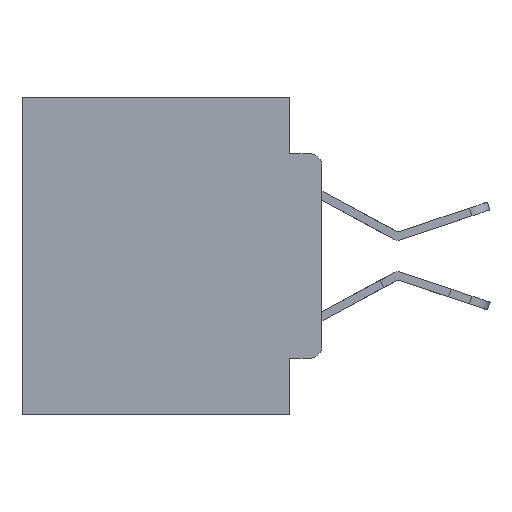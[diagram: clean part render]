
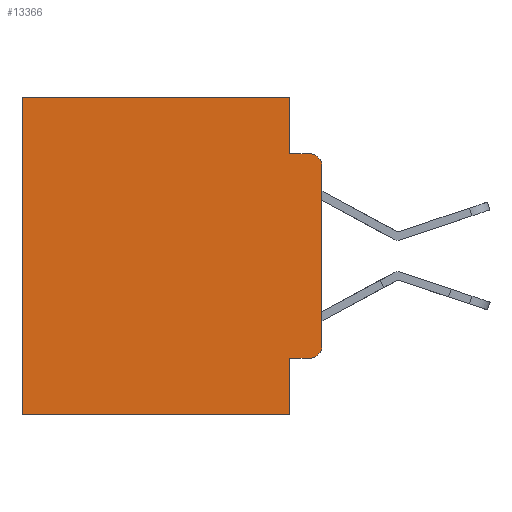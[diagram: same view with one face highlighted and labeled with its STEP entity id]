
A CAD part, left-side view. The second image highlights one B-rep face of the part: STEP entity #13366.
In plain terms, the highlighted planar face has unit normal (-1, 0, 0).
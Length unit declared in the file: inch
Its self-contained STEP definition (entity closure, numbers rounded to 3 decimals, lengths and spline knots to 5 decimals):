
#502 = LINE ( 'NONE', #6662, #24022 ) ;
#746 = VECTOR ( 'NONE', #17544, 39.37008 ) ;
#786 = CARTESIAN_POINT ( 'NONE',  ( 0.298, 0., -0.1085 ) ) ;
#980 = VERTEX_POINT ( 'NONE', #29795 ) ;
#1310 = EDGE_CURVE ( 'NONE', #6025, #29234, #16941, .T. ) ;
#1388 = DIRECTION ( 'NONE',  ( 0., 0., -1. ) ) ;
#1854 = LINE ( 'NONE', #29069, #21708 ) ;
#2882 = ORIENTED_EDGE ( 'NONE', *, *, #23041, .F. ) ;
#2899 = DIRECTION ( 'NONE',  ( 0., 0., -1. ) ) ;
#2971 = CARTESIAN_POINT ( 'NONE',  ( 0.298, 0.02, -0.1085 ) ) ;
#3745 = LINE ( 'NONE', #8295, #15320 ) ;
#3854 = PLANE ( 'NONE',  #16851 ) ;
#4271 = VERTEX_POINT ( 'NONE', #22467 ) ;
#4990 = DIRECTION ( 'NONE',  ( 0., -1., 0. ) ) ;
#5420 = VECTOR ( 'NONE', #11482, 39.37008 ) ;
#5625 = FACE_OUTER_BOUND ( 'NONE', #14080, .T. ) ;
#5909 = CARTESIAN_POINT ( 'NONE',  ( 0.298, 0., -0.5 ) ) ;
#6025 = VERTEX_POINT ( 'NONE', #17912 ) ;
#6082 = DIRECTION ( 'NONE',  ( -1., 0., 0. ) ) ;
#6245 = DIRECTION ( 'NONE',  ( 0., 0., -1. ) ) ;
#6429 = EDGE_CURVE ( 'NONE', #980, #21504, #19172, .T. ) ;
#6631 = EDGE_CURVE ( 'NONE', #27518, #980, #18816, .T. ) ;
#6662 = CARTESIAN_POINT ( 'NONE',  ( 0.298, 0., 0. ) ) ;
#7044 = EDGE_CURVE ( 'NONE', #4271, #11649, #13814, .T. ) ;
#7847 = ORIENTED_EDGE ( 'NONE', *, *, #16300, .F. ) ;
#8295 = CARTESIAN_POINT ( 'NONE',  ( 0.298, 0., 0. ) ) ;
#8607 = EDGE_CURVE ( 'NONE', #27518, #4271, #1854, .T. ) ;
#8631 = CARTESIAN_POINT ( 'NONE',  ( 0.298, 0.02, -0.3915 ) ) ;
#8725 = CARTESIAN_POINT ( 'NONE',  ( 0.298, 0., -0.3915 ) ) ;
#9327 = CARTESIAN_POINT ( 'NONE',  ( 0.298, 0.473, 0. ) ) ;
#10028 = ORIENTED_EDGE ( 'NONE', *, *, #6631, .F. ) ;
#10473 = VECTOR ( 'NONE', #4990, 39.37008 ) ;
#10656 = ORIENTED_EDGE ( 'NONE', *, *, #1310, .F. ) ;
#10748 = CARTESIAN_POINT ( 'NONE',  ( 0.298, 0.473, 0. ) ) ;
#10967 = LINE ( 'NONE', #21297, #21469 ) ;
#11482 = DIRECTION ( 'NONE',  ( 0., 0., -1. ) ) ;
#11649 = VERTEX_POINT ( 'NONE', #8725 ) ;
#11676 = CARTESIAN_POINT ( 'NONE',  ( 0.298, 0.051, 0. ) ) ;
#11955 = CARTESIAN_POINT ( 'NONE',  ( 0.298, 0.051, -0.0885 ) ) ;
#12788 = ORIENTED_EDGE ( 'NONE', *, *, #23403, .T. ) ;
#13366 = ADVANCED_FACE ( 'NONE', ( #5625 ), #3854, .F. ) ;
#13814 = CIRCLE ( 'NONE', #14035, 0.02 ) ;
#14035 = AXIS2_PLACEMENT_3D ( 'NONE', #8631, #6082, #26933 ) ;
#14080 = EDGE_LOOP ( 'NONE', ( #7847, #21992, #10656, #2882, #15908, #12788, #27070, #10028, #16103, #24958 ) ) ;
#14281 = DIRECTION ( 'NONE',  ( 0., 0., -1. ) ) ;
#14675 = CARTESIAN_POINT ( 'NONE',  ( 0.298, 0.051, -0.4115 ) ) ;
#15066 = DIRECTION ( 'NONE',  ( 0., 0., -1. ) ) ;
#15320 = VECTOR ( 'NONE', #15066, 39.37008 ) ;
#15389 = EDGE_CURVE ( 'NONE', #29398, #25611, #502, .T. ) ;
#15908 = ORIENTED_EDGE ( 'NONE', *, *, #15389, .T. ) ;
#16103 = ORIENTED_EDGE ( 'NONE', *, *, #8607, .T. ) ;
#16300 = EDGE_CURVE ( 'NONE', #18913, #11649, #3745, .T. ) ;
#16816 = CARTESIAN_POINT ( 'NONE',  ( 0.298, 0.473, -0.5 ) ) ;
#16824 = AXIS2_PLACEMENT_3D ( 'NONE', #2971, #23864, #14281 ) ;
#16851 = AXIS2_PLACEMENT_3D ( 'NONE', #20009, #29133, #6245 ) ;
#16941 = LINE ( 'NONE', #11955, #10473 ) ;
#17544 = DIRECTION ( 'NONE',  ( 0., 1., 0. ) ) ;
#17912 = CARTESIAN_POINT ( 'NONE',  ( 0.298, 0.051, -0.0885 ) ) ;
#18816 = LINE ( 'NONE', #11676, #5420 ) ;
#18913 = VERTEX_POINT ( 'NONE', #786 ) ;
#19172 = LINE ( 'NONE', #5909, #746 ) ;
#20009 = CARTESIAN_POINT ( 'NONE',  ( 0.298, 0., 0. ) ) ;
#21297 = CARTESIAN_POINT ( 'NONE',  ( 0.298, 0.051, 0. ) ) ;
#21469 = VECTOR ( 'NONE', #2899, 39.37008 ) ;
#21504 = VERTEX_POINT ( 'NONE', #16816 ) ;
#21607 = CARTESIAN_POINT ( 'NONE',  ( 0.298, 0.02, -0.0885 ) ) ;
#21708 = VECTOR ( 'NONE', #28760, 39.37008 ) ;
#21992 = ORIENTED_EDGE ( 'NONE', *, *, #28479, .T. ) ;
#22467 = CARTESIAN_POINT ( 'NONE',  ( 0.298, 0.02, -0.4115 ) ) ;
#23041 = EDGE_CURVE ( 'NONE', #29398, #6025, #10967, .T. ) ;
#23389 = CIRCLE ( 'NONE', #16824, 0.02 ) ;
#23403 = EDGE_CURVE ( 'NONE', #25611, #21504, #28319, .T. ) ;
#23864 = DIRECTION ( 'NONE',  ( -1., 0., 0. ) ) ;
#24022 = VECTOR ( 'NONE', #27522, 39.37008 ) ;
#24681 = VECTOR ( 'NONE', #1388, 39.37008 ) ;
#24958 = ORIENTED_EDGE ( 'NONE', *, *, #7044, .T. ) ;
#25611 = VERTEX_POINT ( 'NONE', #9327 ) ;
#26933 = DIRECTION ( 'NONE',  ( 0., 0., -1. ) ) ;
#27070 = ORIENTED_EDGE ( 'NONE', *, *, #6429, .F. ) ;
#27375 = CARTESIAN_POINT ( 'NONE',  ( 0.298, 0.051, 0. ) ) ;
#27518 = VERTEX_POINT ( 'NONE', #14675 ) ;
#27522 = DIRECTION ( 'NONE',  ( 0., 1., 0. ) ) ;
#28319 = LINE ( 'NONE', #10748, #24681 ) ;
#28479 = EDGE_CURVE ( 'NONE', #18913, #29234, #23389, .T. ) ;
#28760 = DIRECTION ( 'NONE',  ( 0., -1., 0. ) ) ;
#29069 = CARTESIAN_POINT ( 'NONE',  ( 0.298, 0.051, -0.4115 ) ) ;
#29133 = DIRECTION ( 'NONE',  ( 1., 0., 0. ) ) ;
#29234 = VERTEX_POINT ( 'NONE', #21607 ) ;
#29398 = VERTEX_POINT ( 'NONE', #27375 ) ;
#29795 = CARTESIAN_POINT ( 'NONE',  ( 0.298, 0.051, -0.5 ) ) ;
